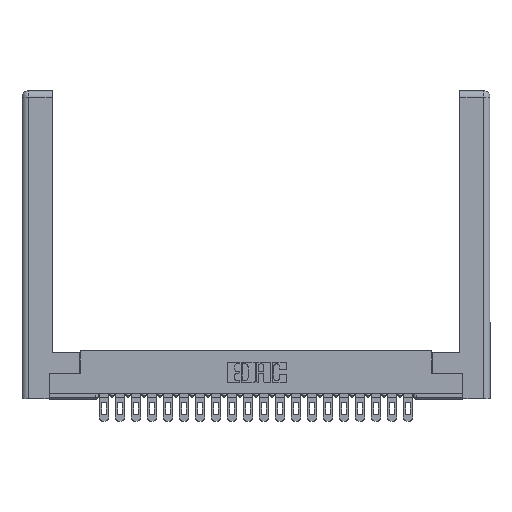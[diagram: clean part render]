
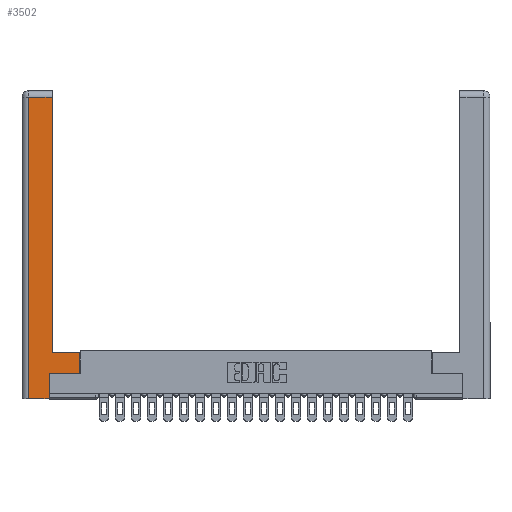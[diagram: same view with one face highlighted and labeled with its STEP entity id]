
A CAD part, top view. The second image highlights one B-rep face of the part: STEP entity #3502.
In plain terms, the highlighted planar face has unit normal (0, 0, 1).
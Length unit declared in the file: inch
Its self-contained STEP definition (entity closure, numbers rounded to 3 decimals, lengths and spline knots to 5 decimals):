
#339 = LINE ( 'NONE', #20570, #18890 ) ;
#427 = DIRECTION ( 'NONE',  ( 0., 0., -1. ) ) ;
#532 = CARTESIAN_POINT ( 'NONE',  ( 0.295, 3., 0. ) ) ;
#1095 = LINE ( 'NONE', #9005, #10098 ) ;
#1742 = ORIENTED_EDGE ( 'NONE', *, *, #10217, .T. ) ;
#2057 = VERTEX_POINT ( 'NONE', #2099 ) ;
#2099 = CARTESIAN_POINT ( 'NONE',  ( 0.565, 0.245, 0. ) ) ;
#2380 = EDGE_CURVE ( 'NONE', #15429, #12416, #3388, .T. ) ;
#2431 = CARTESIAN_POINT ( 'NONE',  ( 0.265, 0.245, 0. ) ) ;
#2502 = DIRECTION ( 'NONE',  ( 1., 0., 0. ) ) ;
#2681 = DIRECTION ( 'NONE',  ( -1., 0., 0. ) ) ;
#3083 = EDGE_CURVE ( 'NONE', #12416, #3147, #22617, .T. ) ;
#3147 = VERTEX_POINT ( 'NONE', #9246 ) ;
#3388 = LINE ( 'NONE', #13459, #8186 ) ;
#3502 = ADVANCED_FACE ( 'NONE', ( #5169 ), #7877, .F. ) ;
#4033 = VERTEX_POINT ( 'NONE', #2431 ) ;
#4750 = EDGE_LOOP ( 'NONE', ( #1742, #14003, #15525, #12293, #6701, #11535, #11957, #11839 ) ) ;
#4757 = LINE ( 'NONE', #532, #7269 ) ;
#4900 = LINE ( 'NONE', #20129, #7989 ) ;
#4947 = LINE ( 'NONE', #22384, #16211 ) ;
#5169 = FACE_OUTER_BOUND ( 'NONE', #4750, .T. ) ;
#5317 = DIRECTION ( 'NONE',  ( 0., -1., 0. ) ) ;
#6007 = CARTESIAN_POINT ( 'NONE',  ( 0., 0., 0. ) ) ;
#6701 = ORIENTED_EDGE ( 'NONE', *, *, #20236, .T. ) ;
#6819 = VERTEX_POINT ( 'NONE', #23205 ) ;
#6886 = CARTESIAN_POINT ( 'NONE',  ( 0.295, 2.94, 0. ) ) ;
#7026 = DIRECTION ( 'NONE',  ( -1., 0., 0. ) ) ;
#7269 = VECTOR ( 'NONE', #15443, 39.37008 ) ;
#7729 = VECTOR ( 'NONE', #5317, 39.37008 ) ;
#7877 = PLANE ( 'NONE',  #21220 ) ;
#7989 = VECTOR ( 'NONE', #20199, 39.37008 ) ;
#8186 = VECTOR ( 'NONE', #2681, 39.37008 ) ;
#9005 = CARTESIAN_POINT ( 'NONE',  ( 0.295, 0.45, 0. ) ) ;
#9246 = CARTESIAN_POINT ( 'NONE',  ( 0.0615, 0., 0. ) ) ;
#9588 = CARTESIAN_POINT ( 'NONE',  ( 0.295, 0.45, 0. ) ) ;
#10039 = CARTESIAN_POINT ( 'NONE',  ( 0.265, 0., 0. ) ) ;
#10098 = VECTOR ( 'NONE', #7026, 39.37008 ) ;
#10217 = EDGE_CURVE ( 'NONE', #18711, #15429, #4757, .T. ) ;
#10238 = VECTOR ( 'NONE', #22727, 39.37008 ) ;
#10551 = EDGE_CURVE ( 'NONE', #6819, #18711, #1095, .T. ) ;
#11535 = ORIENTED_EDGE ( 'NONE', *, *, #19116, .T. ) ;
#11632 = LINE ( 'NONE', #21030, #10238 ) ;
#11839 = ORIENTED_EDGE ( 'NONE', *, *, #10551, .T. ) ;
#11957 = ORIENTED_EDGE ( 'NONE', *, *, #22950, .T. ) ;
#12293 = ORIENTED_EDGE ( 'NONE', *, *, #21050, .T. ) ;
#12416 = VERTEX_POINT ( 'NONE', #16548 ) ;
#13459 = CARTESIAN_POINT ( 'NONE',  ( 0.0615, 2.94, 0. ) ) ;
#14003 = ORIENTED_EDGE ( 'NONE', *, *, #2380, .T. ) ;
#15429 = VERTEX_POINT ( 'NONE', #6886 ) ;
#15443 = DIRECTION ( 'NONE',  ( 0., 1., 0. ) ) ;
#15525 = ORIENTED_EDGE ( 'NONE', *, *, #3083, .T. ) ;
#16211 = VECTOR ( 'NONE', #2502, 39.37008 ) ;
#16548 = CARTESIAN_POINT ( 'NONE',  ( 0.0615, 2.94, 0. ) ) ;
#16691 = DIRECTION ( 'NONE',  ( -1., 0., 0. ) ) ;
#18133 = CARTESIAN_POINT ( 'NONE',  ( 0.0615, 0., 0. ) ) ;
#18711 = VERTEX_POINT ( 'NONE', #9588 ) ;
#18833 = DIRECTION ( 'NONE',  ( 1., 0., 0. ) ) ;
#18890 = VECTOR ( 'NONE', #18833, 39.37008 ) ;
#19116 = EDGE_CURVE ( 'NONE', #4033, #2057, #4947, .T. ) ;
#20129 = CARTESIAN_POINT ( 'NONE',  ( 0.265, 0.245, 0. ) ) ;
#20199 = DIRECTION ( 'NONE',  ( 0., 1., 0. ) ) ;
#20236 = EDGE_CURVE ( 'NONE', #21652, #4033, #4900, .T. ) ;
#20570 = CARTESIAN_POINT ( 'NONE',  ( 0.265, 0., 0. ) ) ;
#21030 = CARTESIAN_POINT ( 'NONE',  ( 0.565, 0.45, 0. ) ) ;
#21050 = EDGE_CURVE ( 'NONE', #3147, #21652, #339, .T. ) ;
#21220 = AXIS2_PLACEMENT_3D ( 'NONE', #6007, #427, #16691 ) ;
#21652 = VERTEX_POINT ( 'NONE', #10039 ) ;
#22384 = CARTESIAN_POINT ( 'NONE',  ( 0.565, 0.245, 0. ) ) ;
#22617 = LINE ( 'NONE', #18133, #7729 ) ;
#22727 = DIRECTION ( 'NONE',  ( 0., 1., 0. ) ) ;
#22950 = EDGE_CURVE ( 'NONE', #2057, #6819, #11632, .T. ) ;
#23205 = CARTESIAN_POINT ( 'NONE',  ( 0.565, 0.45, 0. ) ) ;
